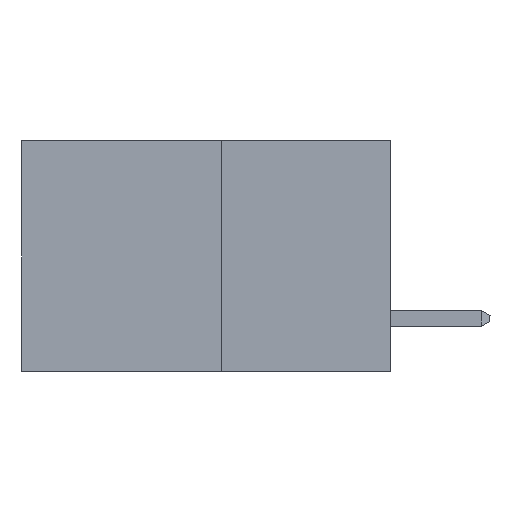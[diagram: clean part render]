
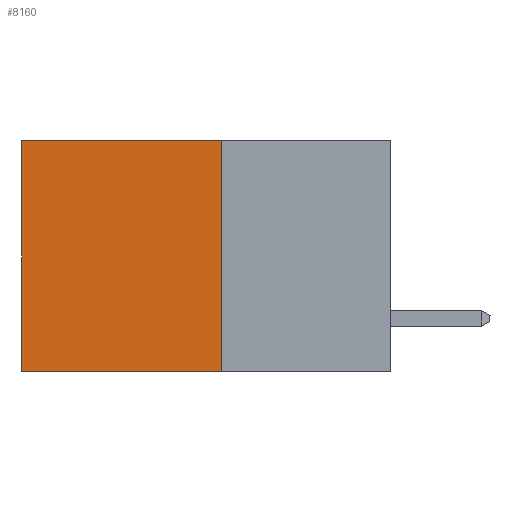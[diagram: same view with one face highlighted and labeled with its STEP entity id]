
A CAD part, left-side view. The second image highlights one B-rep face of the part: STEP entity #8160.
In plain terms, the highlighted planar face has unit normal (-1, 0, 0).
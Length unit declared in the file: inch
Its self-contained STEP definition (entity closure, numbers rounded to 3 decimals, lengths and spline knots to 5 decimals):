
#371 = EDGE_CURVE ( 'NONE', #17406, #7449, #526, .T. ) ;
#526 = LINE ( 'NONE', #8769, #6835 ) ;
#1552 = EDGE_CURVE ( 'NONE', #12909, #17406, #17919, .T. ) ;
#1598 = AXIS2_PLACEMENT_3D ( 'NONE', #8991, #13641, #4352 ) ;
#2215 = CARTESIAN_POINT ( 'NONE',  ( 0.277, 0.27, 0. ) ) ;
#2342 = VERTEX_POINT ( 'NONE', #14480 ) ;
#2579 = VECTOR ( 'NONE', #4213, 39.37008 ) ;
#3129 = EDGE_CURVE ( 'NONE', #12909, #2342, #10101, .T. ) ;
#3285 = EDGE_CURVE ( 'NONE', #2342, #7449, #19970, .T. ) ;
#4213 = DIRECTION ( 'NONE',  ( 0., 1., 0. ) ) ;
#4308 = CARTESIAN_POINT ( 'NONE',  ( 0.277, 0.59, -0.37 ) ) ;
#4352 = DIRECTION ( 'NONE',  ( 0., 0., -1. ) ) ;
#5832 = ORIENTED_EDGE ( 'NONE', *, *, #1552, .T. ) ;
#5853 = PLANE ( 'NONE',  #1598 ) ;
#6207 = ORIENTED_EDGE ( 'NONE', *, *, #3129, .F. ) ;
#6835 = VECTOR ( 'NONE', #18239, 39.37008 ) ;
#6886 = DIRECTION ( 'NONE',  ( 0., 1., 0. ) ) ;
#7272 = CARTESIAN_POINT ( 'NONE',  ( 0.277, 0.27, 0. ) ) ;
#7449 = VERTEX_POINT ( 'NONE', #4308 ) ;
#7911 = CARTESIAN_POINT ( 'NONE',  ( 0.277, 0.59, 0. ) ) ;
#8160 = ADVANCED_FACE ( 'NONE', ( #12577 ), #5853, .F. ) ;
#8769 = CARTESIAN_POINT ( 'NONE',  ( 0.277, 0.59, -0.37 ) ) ;
#8991 = CARTESIAN_POINT ( 'NONE',  ( 0.277, 0.27, -0.37 ) ) ;
#9128 = EDGE_LOOP ( 'NONE', ( #15941, #13519, #6207, #5832 ) ) ;
#9633 = VECTOR ( 'NONE', #17548, 39.37008 ) ;
#10101 = LINE ( 'NONE', #17340, #9633 ) ;
#12577 = FACE_OUTER_BOUND ( 'NONE', #9128, .T. ) ;
#12909 = VERTEX_POINT ( 'NONE', #2215 ) ;
#13519 = ORIENTED_EDGE ( 'NONE', *, *, #3285, .F. ) ;
#13641 = DIRECTION ( 'NONE',  ( 1., 0., 0. ) ) ;
#13799 = VECTOR ( 'NONE', #6886, 39.37008 ) ;
#14306 = CARTESIAN_POINT ( 'NONE',  ( 0.277, 0.27, -0.37 ) ) ;
#14480 = CARTESIAN_POINT ( 'NONE',  ( 0.277, 0.27, -0.37 ) ) ;
#15941 = ORIENTED_EDGE ( 'NONE', *, *, #371, .T. ) ;
#17340 = CARTESIAN_POINT ( 'NONE',  ( 0.277, 0.27, -0.37 ) ) ;
#17406 = VERTEX_POINT ( 'NONE', #7911 ) ;
#17548 = DIRECTION ( 'NONE',  ( 0., 0., -1. ) ) ;
#17919 = LINE ( 'NONE', #7272, #13799 ) ;
#18239 = DIRECTION ( 'NONE',  ( 0., 0., -1. ) ) ;
#19970 = LINE ( 'NONE', #14306, #2579 ) ;
